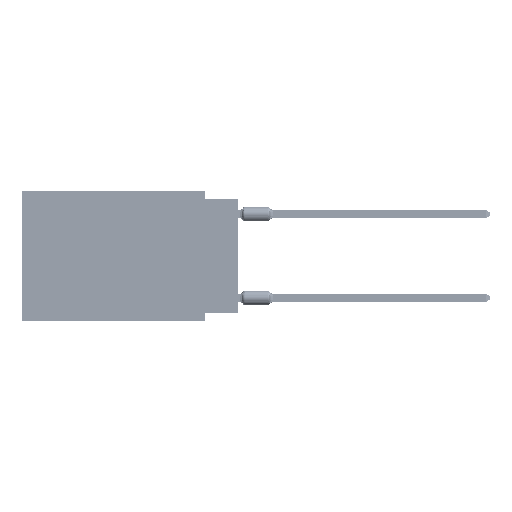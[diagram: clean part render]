
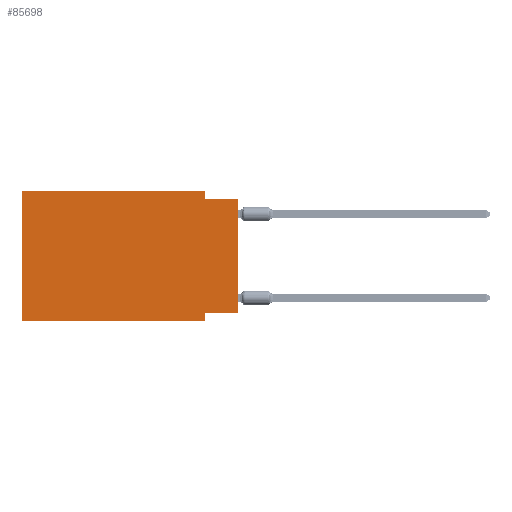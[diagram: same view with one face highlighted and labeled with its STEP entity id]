
A CAD part, left-side view. The second image highlights one B-rep face of the part: STEP entity #85698.
In plain terms, the highlighted planar face has unit normal (-1, 0, 0).
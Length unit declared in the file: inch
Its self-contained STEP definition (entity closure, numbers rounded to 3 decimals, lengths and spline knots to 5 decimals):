
#1809 = DIRECTION ( 'NONE',  ( 0., 0., -1. ) ) ;
#3295 = AXIS2_PLACEMENT_3D ( 'NONE', #63226, #76684, #1809 ) ;
#3616 = VERTEX_POINT ( 'NONE', #61459 ) ;
#3864 = LINE ( 'NONE', #31205, #71049 ) ;
#6695 = EDGE_CURVE ( 'NONE', #39670, #10791, #17220, .T. ) ;
#10791 = VERTEX_POINT ( 'NONE', #81659 ) ;
#10799 = CARTESIAN_POINT ( 'NONE',  ( 0., 0., -0.025 ) ) ;
#11143 = CARTESIAN_POINT ( 'NONE',  ( 0., 0., -0.365 ) ) ;
#11160 = EDGE_LOOP ( 'NONE', ( #32709, #36014, #64954, #69822, #78713, #59499, #86112, #69950 ) ) ;
#12846 = CARTESIAN_POINT ( 'NONE',  ( 0., 0.1, -0.365 ) ) ;
#13284 = VERTEX_POINT ( 'NONE', #11143 ) ;
#13333 = VECTOR ( 'NONE', #67661, 39.37008 ) ;
#13505 = LINE ( 'NONE', #14837, #70904 ) ;
#13840 = LINE ( 'NONE', #81121, #13333 ) ;
#14837 = CARTESIAN_POINT ( 'NONE',  ( 0., 0., -0.365 ) ) ;
#16704 = LINE ( 'NONE', #44058, #61243 ) ;
#17220 = LINE ( 'NONE', #29349, #28770 ) ;
#20550 = VECTOR ( 'NONE', #87134, 39.37008 ) ;
#20573 = DIRECTION ( 'NONE',  ( 0., 0., -1. ) ) ;
#20673 = DIRECTION ( 'NONE',  ( 0., 1., 0. ) ) ;
#21952 = VERTEX_POINT ( 'NONE', #10799 ) ;
#22888 = EDGE_CURVE ( 'NONE', #3616, #39670, #3864, .T. ) ;
#24313 = CARTESIAN_POINT ( 'NONE',  ( 0., 0.1, -0.025 ) ) ;
#28226 = CARTESIAN_POINT ( 'NONE',  ( 0., 0., 0. ) ) ;
#28770 = VECTOR ( 'NONE', #31120, 39.37008 ) ;
#29349 = CARTESIAN_POINT ( 'NONE',  ( 0., 0.645, 0. ) ) ;
#31120 = DIRECTION ( 'NONE',  ( 0., -1., 0. ) ) ;
#31205 = CARTESIAN_POINT ( 'NONE',  ( 0., 0.645, 0. ) ) ;
#31635 = DIRECTION ( 'NONE',  ( 0., 0., 1. ) ) ;
#32330 = PLANE ( 'NONE',  #3295 ) ;
#32709 = ORIENTED_EDGE ( 'NONE', *, *, #84517, .T. ) ;
#36014 = ORIENTED_EDGE ( 'NONE', *, *, #75359, .F. ) ;
#36568 = VERTEX_POINT ( 'NONE', #24313 ) ;
#37040 = EDGE_CURVE ( 'NONE', #74488, #45069, #13840, .T. ) ;
#38671 = CARTESIAN_POINT ( 'NONE',  ( 0., 0., -0.025 ) ) ;
#39670 = VERTEX_POINT ( 'NONE', #78421 ) ;
#41123 = EDGE_CURVE ( 'NONE', #13284, #74488, #13505, .T. ) ;
#44058 = CARTESIAN_POINT ( 'NONE',  ( 0., 0.645, -0.39 ) ) ;
#45069 = VERTEX_POINT ( 'NONE', #84888 ) ;
#47062 = EDGE_CURVE ( 'NONE', #10791, #36568, #60062, .T. ) ;
#55071 = CARTESIAN_POINT ( 'NONE',  ( 0., 0.1, 0. ) ) ;
#59499 = ORIENTED_EDGE ( 'NONE', *, *, #62115, .T. ) ;
#60062 = LINE ( 'NONE', #55071, #79968 ) ;
#61243 = VECTOR ( 'NONE', #71407, 39.37008 ) ;
#61459 = CARTESIAN_POINT ( 'NONE',  ( 0., 0.645, -0.39 ) ) ;
#62115 = EDGE_CURVE ( 'NONE', #3616, #45069, #16704, .T. ) ;
#62324 = LINE ( 'NONE', #28226, #63520 ) ;
#63226 = CARTESIAN_POINT ( 'NONE',  ( 0., 0.645, 0. ) ) ;
#63520 = VECTOR ( 'NONE', #75765, 39.37008 ) ;
#64954 = ORIENTED_EDGE ( 'NONE', *, *, #47062, .F. ) ;
#66415 = FACE_OUTER_BOUND ( 'NONE', #11160, .T. ) ;
#67661 = DIRECTION ( 'NONE',  ( 0., 0., -1. ) ) ;
#69822 = ORIENTED_EDGE ( 'NONE', *, *, #6695, .F. ) ;
#69950 = ORIENTED_EDGE ( 'NONE', *, *, #41123, .F. ) ;
#70904 = VECTOR ( 'NONE', #20673, 39.37008 ) ;
#71049 = VECTOR ( 'NONE', #31635, 39.37008 ) ;
#71407 = DIRECTION ( 'NONE',  ( 0., -1., 0. ) ) ;
#74488 = VERTEX_POINT ( 'NONE', #12846 ) ;
#75359 = EDGE_CURVE ( 'NONE', #36568, #21952, #86687, .T. ) ;
#75765 = DIRECTION ( 'NONE',  ( 0., 0., 1. ) ) ;
#76684 = DIRECTION ( 'NONE',  ( 1., 0., 0. ) ) ;
#78421 = CARTESIAN_POINT ( 'NONE',  ( 0., 0.645, 0. ) ) ;
#78713 = ORIENTED_EDGE ( 'NONE', *, *, #22888, .F. ) ;
#79968 = VECTOR ( 'NONE', #20573, 39.37008 ) ;
#81121 = CARTESIAN_POINT ( 'NONE',  ( 0., 0.1, -0.39 ) ) ;
#81659 = CARTESIAN_POINT ( 'NONE',  ( 0., 0.1, 0. ) ) ;
#84517 = EDGE_CURVE ( 'NONE', #13284, #21952, #62324, .T. ) ;
#84888 = CARTESIAN_POINT ( 'NONE',  ( 0., 0.1, -0.39 ) ) ;
#85698 = ADVANCED_FACE ( 'NONE', ( #66415 ), #32330, .F. ) ;
#86112 = ORIENTED_EDGE ( 'NONE', *, *, #37040, .F. ) ;
#86687 = LINE ( 'NONE', #38671, #20550 ) ;
#87134 = DIRECTION ( 'NONE',  ( 0., -1., 0. ) ) ;
